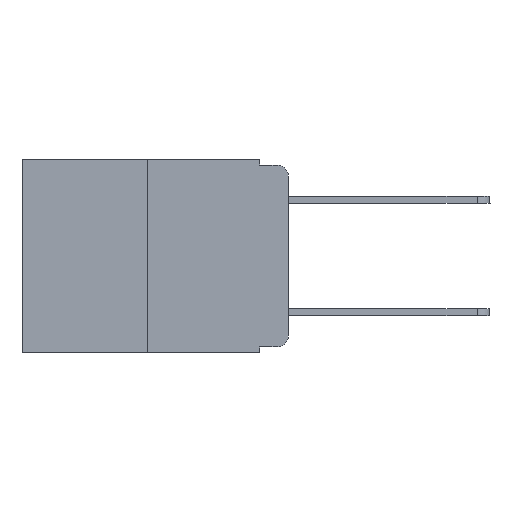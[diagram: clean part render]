
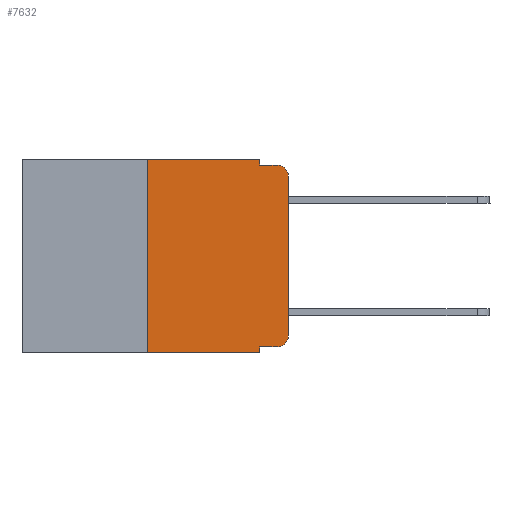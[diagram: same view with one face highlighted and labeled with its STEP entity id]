
A CAD part, left-side view. The second image highlights one B-rep face of the part: STEP entity #7632.
In plain terms, the highlighted planar face has unit normal (-1, 0, 0).
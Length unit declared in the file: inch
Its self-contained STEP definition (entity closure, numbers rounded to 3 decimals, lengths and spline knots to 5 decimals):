
#346 = DIRECTION ( 'NONE',  ( -1., 0., 0. ) ) ;
#362 = CARTESIAN_POINT ( 'NONE',  ( 0., 0.02, -0.01 ) ) ;
#443 = EDGE_CURVE ( 'NONE', #3179, #762, #2282, .T. ) ;
#590 = EDGE_CURVE ( 'NONE', #5566, #3179, #6340, .T. ) ;
#762 = VERTEX_POINT ( 'NONE', #1992 ) ;
#929 = DIRECTION ( 'NONE',  ( 0., -1., 0. ) ) ;
#1148 = EDGE_CURVE ( 'NONE', #7001, #1338, #7900, .T. ) ;
#1166 = DIRECTION ( 'NONE',  ( -1., 0., 0. ) ) ;
#1188 = CARTESIAN_POINT ( 'NONE',  ( 0., 0.051, -0.333 ) ) ;
#1194 = PLANE ( 'NONE',  #4152 ) ;
#1338 = VERTEX_POINT ( 'NONE', #362 ) ;
#1527 = EDGE_CURVE ( 'NONE', #3662, #10540, #10840, .T. ) ;
#1796 = CARTESIAN_POINT ( 'NONE',  ( 0., 0.02, -0.333 ) ) ;
#1958 = CARTESIAN_POINT ( 'NONE',  ( 0., 0.051, -0.01 ) ) ;
#1992 = CARTESIAN_POINT ( 'NONE',  ( 0., 0., -0.313 ) ) ;
#2021 = EDGE_CURVE ( 'NONE', #3097, #1338, #4971, .T. ) ;
#2042 = EDGE_CURVE ( 'NONE', #5566, #10540, #7744, .T. ) ;
#2217 = ORIENTED_EDGE ( 'NONE', *, *, #443, .T. ) ;
#2282 = CIRCLE ( 'NONE', #4484, 0.02 ) ;
#2341 = VECTOR ( 'NONE', #5783, 39.37008 ) ;
#2676 = VECTOR ( 'NONE', #11950, 39.37008 ) ;
#2812 = CARTESIAN_POINT ( 'NONE',  ( 0., 0.051, 0. ) ) ;
#2871 = DIRECTION ( 'NONE',  ( 0., 0., 1. ) ) ;
#3027 = ORIENTED_EDGE ( 'NONE', *, *, #2042, .F. ) ;
#3097 = VERTEX_POINT ( 'NONE', #3321 ) ;
#3162 = CARTESIAN_POINT ( 'NONE',  ( 0., 0.051, -0.343 ) ) ;
#3179 = VERTEX_POINT ( 'NONE', #1796 ) ;
#3217 = DIRECTION ( 'NONE',  ( 1., 0., 0. ) ) ;
#3321 = CARTESIAN_POINT ( 'NONE',  ( 0., 0., -0.03 ) ) ;
#3662 = VERTEX_POINT ( 'NONE', #9358 ) ;
#4076 = ORIENTED_EDGE ( 'NONE', *, *, #1527, .T. ) ;
#4152 = AXIS2_PLACEMENT_3D ( 'NONE', #7190, #3217, #9971 ) ;
#4268 = CARTESIAN_POINT ( 'NONE',  ( 0., 0.051, 0. ) ) ;
#4484 = AXIS2_PLACEMENT_3D ( 'NONE', #9013, #346, #6991 ) ;
#4608 = EDGE_LOOP ( 'NONE', ( #9354, #5289, #6607, #10878, #9872, #11100, #4076, #3027, #12401, #2217 ) ) ;
#4764 = CARTESIAN_POINT ( 'NONE',  ( 0., 0., 0. ) ) ;
#4767 = CARTESIAN_POINT ( 'NONE',  ( 0., 0.02, -0.03 ) ) ;
#4929 = CARTESIAN_POINT ( 'NONE',  ( 0., 0.051, 0. ) ) ;
#4971 = CIRCLE ( 'NONE', #6790, 0.02 ) ;
#5169 = VECTOR ( 'NONE', #2871, 39.37008 ) ;
#5289 = ORIENTED_EDGE ( 'NONE', *, *, #2021, .T. ) ;
#5328 = VERTEX_POINT ( 'NONE', #10609 ) ;
#5566 = VERTEX_POINT ( 'NONE', #1188 ) ;
#5589 = DIRECTION ( 'NONE',  ( 0., -1., 0. ) ) ;
#5618 = DIRECTION ( 'NONE',  ( 0., 0., 1. ) ) ;
#5656 = CARTESIAN_POINT ( 'NONE',  ( 0., 0.051, -0.333 ) ) ;
#5783 = DIRECTION ( 'NONE',  ( 0., 0., -1. ) ) ;
#6019 = LINE ( 'NONE', #10930, #8631 ) ;
#6117 = FACE_OUTER_BOUND ( 'NONE', #4608, .T. ) ;
#6288 = EDGE_CURVE ( 'NONE', #762, #3097, #7684, .T. ) ;
#6340 = LINE ( 'NONE', #5656, #10971 ) ;
#6607 = ORIENTED_EDGE ( 'NONE', *, *, #1148, .F. ) ;
#6790 = AXIS2_PLACEMENT_3D ( 'NONE', #4767, #1166, #8881 ) ;
#6991 = DIRECTION ( 'NONE',  ( 0., 0., -1. ) ) ;
#7001 = VERTEX_POINT ( 'NONE', #7186 ) ;
#7096 = VECTOR ( 'NONE', #929, 39.37008 ) ;
#7186 = CARTESIAN_POINT ( 'NONE',  ( 0., 0.051, -0.01 ) ) ;
#7190 = CARTESIAN_POINT ( 'NONE',  ( 0., 0.473, 0. ) ) ;
#7632 = ADVANCED_FACE ( 'NONE', ( #6117 ), #1194, .F. ) ;
#7644 = LINE ( 'NONE', #9409, #10443 ) ;
#7684 = LINE ( 'NONE', #4764, #5169 ) ;
#7744 = LINE ( 'NONE', #2812, #2341 ) ;
#7760 = CARTESIAN_POINT ( 'NONE',  ( 0., 0.473, -0.343 ) ) ;
#7900 = LINE ( 'NONE', #1958, #10178 ) ;
#7957 = DIRECTION ( 'NONE',  ( 0., -1., 0. ) ) ;
#8631 = VECTOR ( 'NONE', #8873, 39.37008 ) ;
#8873 = DIRECTION ( 'NONE',  ( 0., -1., 0. ) ) ;
#8881 = DIRECTION ( 'NONE',  ( 0., 0., -1. ) ) ;
#9013 = CARTESIAN_POINT ( 'NONE',  ( 0., 0.02, -0.313 ) ) ;
#9304 = EDGE_CURVE ( 'NONE', #10613, #7001, #10086, .T. ) ;
#9354 = ORIENTED_EDGE ( 'NONE', *, *, #6288, .T. ) ;
#9358 = CARTESIAN_POINT ( 'NONE',  ( 0., 0.25, -0.343 ) ) ;
#9409 = CARTESIAN_POINT ( 'NONE',  ( 0., 0.25, 0. ) ) ;
#9872 = ORIENTED_EDGE ( 'NONE', *, *, #10175, .F. ) ;
#9971 = DIRECTION ( 'NONE',  ( 0., 0., -1. ) ) ;
#10086 = LINE ( 'NONE', #4268, #2676 ) ;
#10175 = EDGE_CURVE ( 'NONE', #5328, #10613, #6019, .T. ) ;
#10178 = VECTOR ( 'NONE', #7957, 39.37008 ) ;
#10443 = VECTOR ( 'NONE', #5618, 39.37008 ) ;
#10540 = VERTEX_POINT ( 'NONE', #3162 ) ;
#10609 = CARTESIAN_POINT ( 'NONE',  ( 0., 0.25, 0. ) ) ;
#10613 = VERTEX_POINT ( 'NONE', #4929 ) ;
#10840 = LINE ( 'NONE', #7760, #7096 ) ;
#10878 = ORIENTED_EDGE ( 'NONE', *, *, #9304, .F. ) ;
#10884 = EDGE_CURVE ( 'NONE', #3662, #5328, #7644, .T. ) ;
#10930 = CARTESIAN_POINT ( 'NONE',  ( 0., 0.473, 0. ) ) ;
#10971 = VECTOR ( 'NONE', #5589, 39.37008 ) ;
#11100 = ORIENTED_EDGE ( 'NONE', *, *, #10884, .F. ) ;
#11950 = DIRECTION ( 'NONE',  ( 0., 0., -1. ) ) ;
#12401 = ORIENTED_EDGE ( 'NONE', *, *, #590, .T. ) ;
